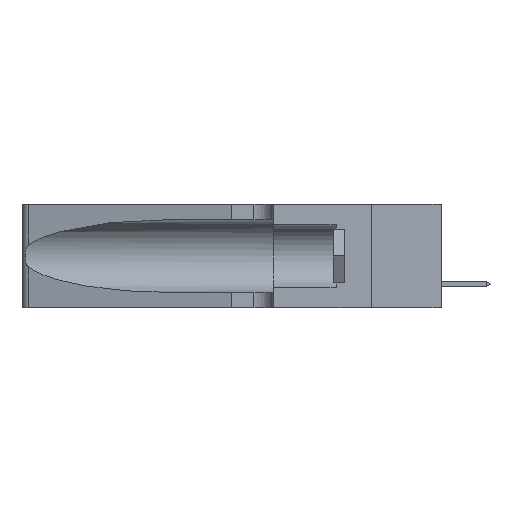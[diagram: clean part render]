
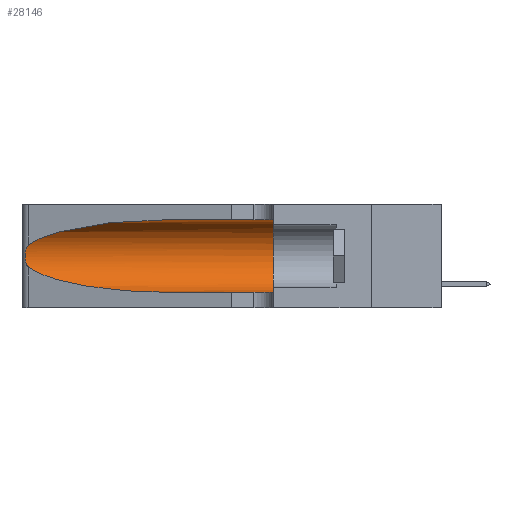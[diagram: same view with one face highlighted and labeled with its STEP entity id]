
A CAD part, left-side view. The second image highlights one B-rep face of the part: STEP entity #28146.
In plain terms, the highlighted cylindrical face has radius 3.308 mm (diameter 6.617 mm), a partial arc.
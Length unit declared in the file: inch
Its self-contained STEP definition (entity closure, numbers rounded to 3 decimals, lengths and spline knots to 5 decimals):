
#510 = EDGE_CURVE ( 'NONE', #14850, #13157, #6797, .T. ) ;
#893 = EDGE_CURVE ( 'NONE', #5902, #14850, #24925, .T. ) ;
#1234 = CARTESIAN_POINT ( 'NONE',  ( 0.1305, 0.72297, 0.31525 ) ) ;
#1807 = CARTESIAN_POINT ( 'NONE',  ( 0.1305, 0.35, 0.31525 ) ) ;
#1945 = ORIENTED_EDGE ( 'NONE', *, *, #27059, .F. ) ;
#2414 = EDGE_CURVE ( 'NONE', #13157, #27507, #28800, .T. ) ;
#2856 = VERTEX_POINT ( 'NONE', #1807 ) ;
#3042 = DIRECTION ( 'NONE',  ( 0., 0., 1. ) ) ;
#3909 = CARTESIAN_POINT ( 'NONE',  ( 0.25555, 1.22993, 0.14849 ) ) ;
#4237 = CARTESIAN_POINT ( 'NONE',  ( 0.25487, 1.22718, 0.22369 ) ) ;
#4494 = CARTESIAN_POINT ( 'NONE',  ( 0.26075, 1.23896, 0.19203 ) ) ;
#4734 = CARTESIAN_POINT ( 'NONE',  ( 0.25487, 1.22718, 0.14631 ) ) ;
#5040 = ORIENTED_EDGE ( 'NONE', *, *, #2414, .T. ) ;
#5068 = VECTOR ( 'NONE', #7600, 39.37008 ) ;
#5127 = CARTESIAN_POINT ( 'NONE',  ( 0.1305, 0.72297, 0.05475 ) ) ;
#5902 = VERTEX_POINT ( 'NONE', #1234 ) ;
#6797 = B_SPLINE_CURVE_WITH_KNOTS ( 'NONE', 3,
 ( #4237, #15568, #7079, #27199, #18731, #21598, #4494, #24459, #7606, #14884, #26284, #11224, #3909, #4734 ),
 .UNSPECIFIED., .F., .F.,
 ( 4, 2, 2, 2, 2, 2, 4 ),
 ( 0., 0.00027, 0.00053, 0.00107, 0.0016, 0.00187, 0.00214 ),
 .UNSPECIFIED. ) ;
#6868 = CARTESIAN_POINT ( 'NONE',  ( 0.25487, 1.22718, 0.14631 ) ) ;
#6872 = DIRECTION ( 'NONE',  ( 0., -1., 0. ) ) ;
#7079 = CARTESIAN_POINT ( 'NONE',  ( 0.25639, 1.23184, 0.21858 ) ) ;
#7188 = CARTESIAN_POINT ( 'NONE',  ( 0.2373, 1.15595, 0.28018 ) ) ;
#7600 = DIRECTION ( 'NONE',  ( 0., -1., 0. ) ) ;
#7606 = CARTESIAN_POINT ( 'NONE',  ( 0.26017, 1.23833, 0.17102 ) ) ;
#8310 = LINE ( 'NONE', #17256, #14101 ) ;
#8853 = CARTESIAN_POINT ( 'NONE',  ( 0.1305, 0.35, 0.185 ) ) ;
#11224 = CARTESIAN_POINT ( 'NONE',  ( 0.25639, 1.23186, 0.15144 ) ) ;
#12457 = ORIENTED_EDGE ( 'NONE', *, *, #13063, .T. ) ;
#12670 = CARTESIAN_POINT ( 'NONE',  ( 0.1305, 0.72297, 0.31525 ) ) ;
#13063 = EDGE_CURVE ( 'NONE', #27507, #22860, #21121, .T. ) ;
#13157 = VERTEX_POINT ( 'NONE', #6868 ) ;
#13211 = CARTESIAN_POINT ( 'NONE',  ( 0.1305, 1.61858, 0.05475 ) ) ;
#14093 = AXIS2_PLACEMENT_3D ( 'NONE', #25849, #29778, #26743 ) ;
#14101 = VECTOR ( 'NONE', #6872, 39.37008 ) ;
#14466 = DIRECTION ( 'NONE',  ( 0., 1., 0. ) ) ;
#14534 = ORIENTED_EDGE ( 'NONE', *, *, #893, .T. ) ;
#14850 = VERTEX_POINT ( 'NONE', #14873 ) ;
#14873 = CARTESIAN_POINT ( 'NONE',  ( 0.25487, 1.22718, 0.22369 ) ) ;
#14884 = CARTESIAN_POINT ( 'NONE',  ( 0.25856, 1.23593, 0.16098 ) ) ;
#15466 = CYLINDRICAL_SURFACE ( 'NONE', #14093, 0.13025 ) ;
#15568 = CARTESIAN_POINT ( 'NONE',  ( 0.25555, 1.22994, 0.2215 ) ) ;
#16330 = CARTESIAN_POINT ( 'NONE',  ( 0.18966, 0.96281, 0.05475 ) ) ;
#17256 = CARTESIAN_POINT ( 'NONE',  ( 0.1305, 1.61858, 0.31525 ) ) ;
#18704 = CARTESIAN_POINT ( 'NONE',  ( 0.25487, 1.22718, 0.22369 ) ) ;
#18731 = CARTESIAN_POINT ( 'NONE',  ( 0.25854, 1.2359, 0.20912 ) ) ;
#20885 = CARTESIAN_POINT ( 'NONE',  ( 0.1305, 0.72297, 0.05475 ) ) ;
#21121 = LINE ( 'NONE', #13211, #5068 ) ;
#21500 = AXIS2_PLACEMENT_3D ( 'NONE', #8853, #14466, #3042 ) ;
#21598 = CARTESIAN_POINT ( 'NONE',  ( 0.26018, 1.23835, 0.19895 ) ) ;
#21658 = EDGE_CURVE ( 'NONE', #5902, #2856, #8310, .T. ) ;
#22860 = VERTEX_POINT ( 'NONE', #24950 ) ;
#24172 = ORIENTED_EDGE ( 'NONE', *, *, #510, .T. ) ;
#24459 = CARTESIAN_POINT ( 'NONE',  ( 0.26075, 1.23896, 0.178 ) ) ;
#24925 =( BOUNDED_CURVE ( )  B_SPLINE_CURVE ( 3, ( #12670, #29959, #7188, #18704 ),
 .UNSPECIFIED., .F., .T. ) 
 B_SPLINE_CURVE_WITH_KNOTS ( ( 4, 4 ),
 ( 1.5708, 2.84003 ),
 .UNSPECIFIED. ) 
 CURVE ( )  GEOMETRIC_REPRESENTATION_ITEM ( )  RATIONAL_B_SPLINE_CURVE ( ( 1., 0.87, 0.87, 1. ) ) 
 REPRESENTATION_ITEM ( '' )  );
#24950 = CARTESIAN_POINT ( 'NONE',  ( 0.1305, 0.35, 0.05475 ) ) ;
#25199 = CARTESIAN_POINT ( 'NONE',  ( 0.25487, 1.22718, 0.14631 ) ) ;
#25849 = CARTESIAN_POINT ( 'NONE',  ( 0.1305, 1.61858, 0.185 ) ) ;
#26284 = CARTESIAN_POINT ( 'NONE',  ( 0.25789, 1.23486, 0.15765 ) ) ;
#26743 = DIRECTION ( 'NONE',  ( 0., 0., -1. ) ) ;
#27059 = EDGE_CURVE ( 'NONE', #2856, #22860, #34418, .T. ) ;
#27199 = CARTESIAN_POINT ( 'NONE',  ( 0.25787, 1.23484, 0.2124 ) ) ;
#27507 = VERTEX_POINT ( 'NONE', #20885 ) ;
#27855 = CARTESIAN_POINT ( 'NONE',  ( 0.2373, 1.15595, 0.08982 ) ) ;
#28146 = ADVANCED_FACE ( 'NONE', ( #28880 ), #15466, .F. ) ;
#28800 =( BOUNDED_CURVE ( )  B_SPLINE_CURVE ( 3, ( #25199, #27855, #16330, #5127 ),
 .UNSPECIFIED., .F., .F. ) 
 B_SPLINE_CURVE_WITH_KNOTS ( ( 4, 4 ),
 ( 3.44316, 4.71239 ),
 .UNSPECIFIED. ) 
 CURVE ( )  GEOMETRIC_REPRESENTATION_ITEM ( )  RATIONAL_B_SPLINE_CURVE ( ( 1., 0.87, 0.87, 1. ) ) 
 REPRESENTATION_ITEM ( '' )  );
#28880 = FACE_OUTER_BOUND ( 'NONE', #35513, .T. ) ;
#29778 = DIRECTION ( 'NONE',  ( 0., -1., 0. ) ) ;
#29959 = CARTESIAN_POINT ( 'NONE',  ( 0.18966, 0.96281, 0.31525 ) ) ;
#33677 = ORIENTED_EDGE ( 'NONE', *, *, #21658, .F. ) ;
#34418 = CIRCLE ( 'NONE', #21500, 0.13025 ) ;
#35513 = EDGE_LOOP ( 'NONE', ( #14534, #24172, #5040, #12457, #1945, #33677 ) ) ;
